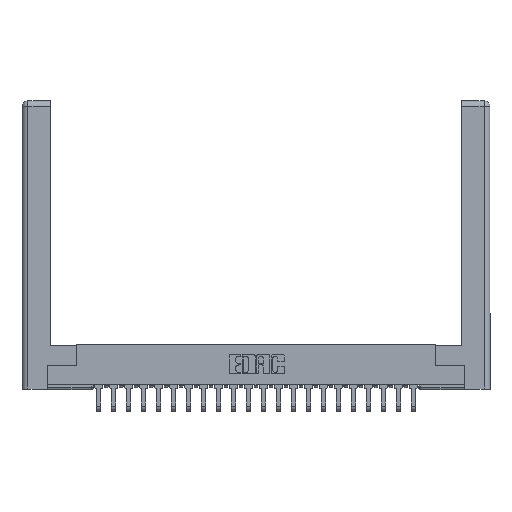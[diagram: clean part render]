
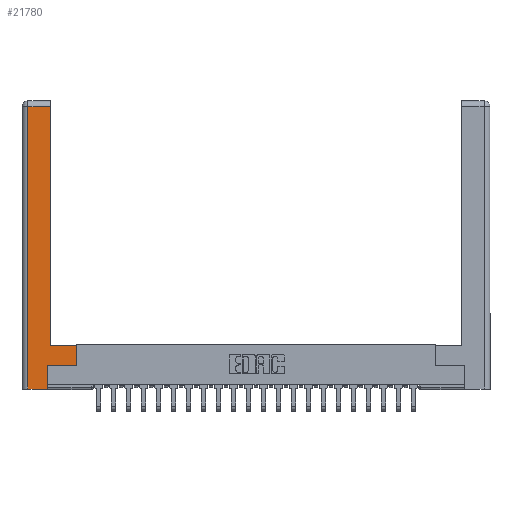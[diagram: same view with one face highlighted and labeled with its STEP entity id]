
A CAD part, top view. The second image highlights one B-rep face of the part: STEP entity #21780.
In plain terms, the highlighted planar face has unit normal (0, 0, 1).
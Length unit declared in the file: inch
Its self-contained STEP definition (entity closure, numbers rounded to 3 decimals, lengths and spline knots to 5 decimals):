
#122 = LINE ( 'NONE', #18363, #13730 ) ;
#1229 = CARTESIAN_POINT ( 'NONE',  ( 0.0615, 0., 0. ) ) ;
#1449 = EDGE_CURVE ( 'NONE', #21751, #6807, #2738, .T. ) ;
#2230 = LINE ( 'NONE', #11742, #11971 ) ;
#2330 = DIRECTION ( 'NONE',  ( -1., 0., 0. ) ) ;
#2601 = CARTESIAN_POINT ( 'NONE',  ( 0.565, 0.45, 0. ) ) ;
#2607 = CARTESIAN_POINT ( 'NONE',  ( 0.265, 0.245, 0. ) ) ;
#2738 = LINE ( 'NONE', #18594, #13274 ) ;
#3608 = FACE_OUTER_BOUND ( 'NONE', #18954, .T. ) ;
#4268 = CARTESIAN_POINT ( 'NONE',  ( 0.295, 2.94, 0. ) ) ;
#4590 = CARTESIAN_POINT ( 'NONE',  ( 0.0615, 0., 0. ) ) ;
#4721 = LINE ( 'NONE', #10780, #17896 ) ;
#6114 = ORIENTED_EDGE ( 'NONE', *, *, #14983, .T. ) ;
#6807 = VERTEX_POINT ( 'NONE', #7125 ) ;
#7125 = CARTESIAN_POINT ( 'NONE',  ( 0.295, 0.45, 0. ) ) ;
#7311 = CARTESIAN_POINT ( 'NONE',  ( 0.565, 0.45, 0. ) ) ;
#7610 = CARTESIAN_POINT ( 'NONE',  ( 0.0615, 2.94, 0. ) ) ;
#8222 = VECTOR ( 'NONE', #16872, 39.37008 ) ;
#9033 = CARTESIAN_POINT ( 'NONE',  ( 0., 0., 0. ) ) ;
#9252 = ORIENTED_EDGE ( 'NONE', *, *, #13680, .T. ) ;
#9538 = VERTEX_POINT ( 'NONE', #17682 ) ;
#9771 = DIRECTION ( 'NONE',  ( 1., 0., 0. ) ) ;
#10028 = CARTESIAN_POINT ( 'NONE',  ( 0.295, 3., 0. ) ) ;
#10502 = VERTEX_POINT ( 'NONE', #4268 ) ;
#10780 = CARTESIAN_POINT ( 'NONE',  ( 0.0615, 2.94, 0. ) ) ;
#10907 = LINE ( 'NONE', #2601, #8222 ) ;
#11742 = CARTESIAN_POINT ( 'NONE',  ( 0.565, 0.245, 0. ) ) ;
#11971 = VECTOR ( 'NONE', #9771, 39.37008 ) ;
#12187 = ORIENTED_EDGE ( 'NONE', *, *, #1449, .T. ) ;
#13112 = EDGE_CURVE ( 'NONE', #9538, #16708, #2230, .T. ) ;
#13274 = VECTOR ( 'NONE', #20691, 39.37008 ) ;
#13631 = CARTESIAN_POINT ( 'NONE',  ( 0.565, 0.245, 0. ) ) ;
#13680 = EDGE_CURVE ( 'NONE', #16708, #21751, #10907, .T. ) ;
#13730 = VECTOR ( 'NONE', #14263, 39.37008 ) ;
#13741 = LINE ( 'NONE', #10028, #16620 ) ;
#14263 = DIRECTION ( 'NONE',  ( 1., 0., 0. ) ) ;
#14983 = EDGE_CURVE ( 'NONE', #17460, #9538, #20824, .T. ) ;
#15096 = VERTEX_POINT ( 'NONE', #4590 ) ;
#15138 = LINE ( 'NONE', #1229, #23516 ) ;
#15559 = EDGE_CURVE ( 'NONE', #24575, #15096, #15138, .T. ) ;
#15876 = VECTOR ( 'NONE', #20417, 39.37008 ) ;
#16419 = AXIS2_PLACEMENT_3D ( 'NONE', #9033, #25161, #19313 ) ;
#16431 = ORIENTED_EDGE ( 'NONE', *, *, #15559, .T. ) ;
#16620 = VECTOR ( 'NONE', #25909, 39.37008 ) ;
#16708 = VERTEX_POINT ( 'NONE', #13631 ) ;
#16770 = CARTESIAN_POINT ( 'NONE',  ( 0.265, 0., 0. ) ) ;
#16872 = DIRECTION ( 'NONE',  ( 0., 1., 0. ) ) ;
#17381 = EDGE_CURVE ( 'NONE', #6807, #10502, #13741, .T. ) ;
#17460 = VERTEX_POINT ( 'NONE', #16770 ) ;
#17490 = DIRECTION ( 'NONE',  ( 0., -1., 0. ) ) ;
#17682 = CARTESIAN_POINT ( 'NONE',  ( 0.265, 0.245, 0. ) ) ;
#17846 = EDGE_CURVE ( 'NONE', #10502, #24575, #4721, .T. ) ;
#17896 = VECTOR ( 'NONE', #2330, 39.37008 ) ;
#18363 = CARTESIAN_POINT ( 'NONE',  ( 0.265, 0., 0. ) ) ;
#18594 = CARTESIAN_POINT ( 'NONE',  ( 0.295, 0.45, 0. ) ) ;
#18653 = EDGE_CURVE ( 'NONE', #15096, #17460, #122, .T. ) ;
#18954 = EDGE_LOOP ( 'NONE', ( #24243, #19100, #16431, #19107, #6114, #24620, #9252, #12187 ) ) ;
#19071 = PLANE ( 'NONE',  #16419 ) ;
#19100 = ORIENTED_EDGE ( 'NONE', *, *, #17846, .T. ) ;
#19107 = ORIENTED_EDGE ( 'NONE', *, *, #18653, .T. ) ;
#19313 = DIRECTION ( 'NONE',  ( -1., 0., 0. ) ) ;
#20417 = DIRECTION ( 'NONE',  ( 0., 1., 0. ) ) ;
#20691 = DIRECTION ( 'NONE',  ( -1., 0., 0. ) ) ;
#20824 = LINE ( 'NONE', #2607, #15876 ) ;
#21751 = VERTEX_POINT ( 'NONE', #7311 ) ;
#21780 = ADVANCED_FACE ( 'NONE', ( #3608 ), #19071, .F. ) ;
#23516 = VECTOR ( 'NONE', #17490, 39.37008 ) ;
#24243 = ORIENTED_EDGE ( 'NONE', *, *, #17381, .T. ) ;
#24575 = VERTEX_POINT ( 'NONE', #7610 ) ;
#24620 = ORIENTED_EDGE ( 'NONE', *, *, #13112, .T. ) ;
#25161 = DIRECTION ( 'NONE',  ( 0., 0., -1. ) ) ;
#25909 = DIRECTION ( 'NONE',  ( 0., 1., 0. ) ) ;
